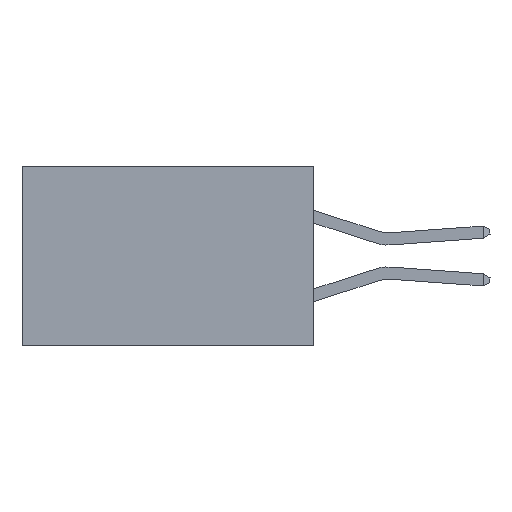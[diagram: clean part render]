
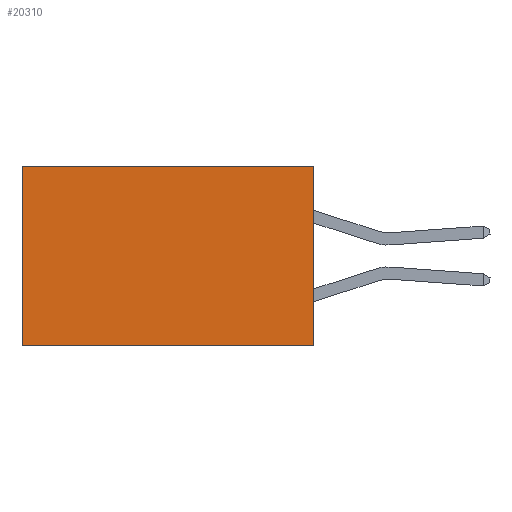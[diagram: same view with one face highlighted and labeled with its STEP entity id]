
A CAD part, left-side view. The second image highlights one B-rep face of the part: STEP entity #20310.
In plain terms, the highlighted planar face has unit normal (-1, 0, 0).
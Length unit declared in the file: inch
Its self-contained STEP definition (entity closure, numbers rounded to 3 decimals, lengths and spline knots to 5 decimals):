
#112 = VERTEX_POINT ( 'NONE', #14226 ) ;
#644 = VECTOR ( 'NONE', #31327, 39.37008 ) ;
#1709 = ORIENTED_EDGE ( 'NONE', *, *, #9521, .F. ) ;
#2139 = DIRECTION ( 'NONE',  ( 0., 0., -1. ) ) ;
#2347 = VECTOR ( 'NONE', #4519, 39.37008 ) ;
#4519 = DIRECTION ( 'NONE',  ( 0., 1., 0. ) ) ;
#4799 = AXIS2_PLACEMENT_3D ( 'NONE', #31596, #18491, #2139 ) ;
#5267 = CARTESIAN_POINT ( 'NONE',  ( 0.2875, 0., -0.37 ) ) ;
#7628 = VECTOR ( 'NONE', #20094, 39.37008 ) ;
#9197 = DIRECTION ( 'NONE',  ( 0., 0., -1. ) ) ;
#9521 = EDGE_CURVE ( 'NONE', #25324, #34338, #14081, .T. ) ;
#9715 = EDGE_CURVE ( 'NONE', #34338, #112, #23166, .T. ) ;
#10357 = PLANE ( 'NONE',  #4799 ) ;
#11309 = ORIENTED_EDGE ( 'NONE', *, *, #13471, .T. ) ;
#13471 = EDGE_CURVE ( 'NONE', #25324, #22582, #23930, .T. ) ;
#14081 = LINE ( 'NONE', #22721, #7628 ) ;
#14226 = CARTESIAN_POINT ( 'NONE',  ( 0.2875, 0.6, -0.37 ) ) ;
#15408 = FACE_OUTER_BOUND ( 'NONE', #24583, .T. ) ;
#15544 = CARTESIAN_POINT ( 'NONE',  ( 0.2875, 0., -0.37 ) ) ;
#15962 = LINE ( 'NONE', #33112, #29169 ) ;
#18491 = DIRECTION ( 'NONE',  ( 1., 0., 0. ) ) ;
#20094 = DIRECTION ( 'NONE',  ( 0., 0., -1. ) ) ;
#20310 = ADVANCED_FACE ( 'NONE', ( #15408 ), #10357, .F. ) ;
#21007 = CARTESIAN_POINT ( 'NONE',  ( 0.2875, 0.6, 0. ) ) ;
#21314 = ORIENTED_EDGE ( 'NONE', *, *, #9715, .F. ) ;
#22014 = CARTESIAN_POINT ( 'NONE',  ( 0.2875, 0., 0. ) ) ;
#22582 = VERTEX_POINT ( 'NONE', #21007 ) ;
#22721 = CARTESIAN_POINT ( 'NONE',  ( 0.2875, 0., 0. ) ) ;
#23166 = LINE ( 'NONE', #15544, #644 ) ;
#23930 = LINE ( 'NONE', #26015, #2347 ) ;
#24583 = EDGE_LOOP ( 'NONE', ( #32166, #21314, #1709, #11309 ) ) ;
#24930 = EDGE_CURVE ( 'NONE', #22582, #112, #15962, .T. ) ;
#25324 = VERTEX_POINT ( 'NONE', #22014 ) ;
#26015 = CARTESIAN_POINT ( 'NONE',  ( 0.2875, 0., 0. ) ) ;
#29169 = VECTOR ( 'NONE', #9197, 39.37008 ) ;
#31327 = DIRECTION ( 'NONE',  ( 0., 1., 0. ) ) ;
#31596 = CARTESIAN_POINT ( 'NONE',  ( 0.2875, 0., 0. ) ) ;
#32166 = ORIENTED_EDGE ( 'NONE', *, *, #24930, .T. ) ;
#33112 = CARTESIAN_POINT ( 'NONE',  ( 0.2875, 0.6, 0. ) ) ;
#34338 = VERTEX_POINT ( 'NONE', #5267 ) ;
